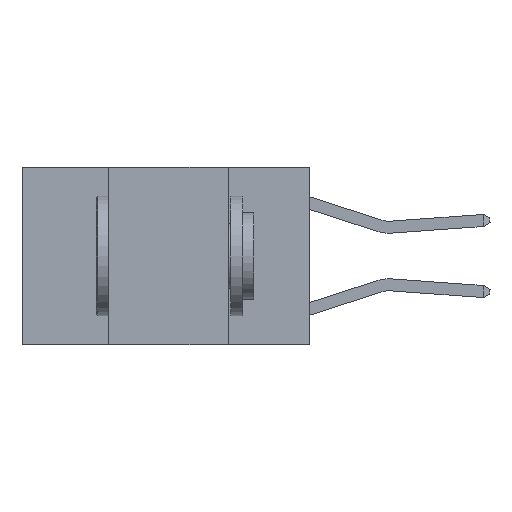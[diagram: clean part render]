
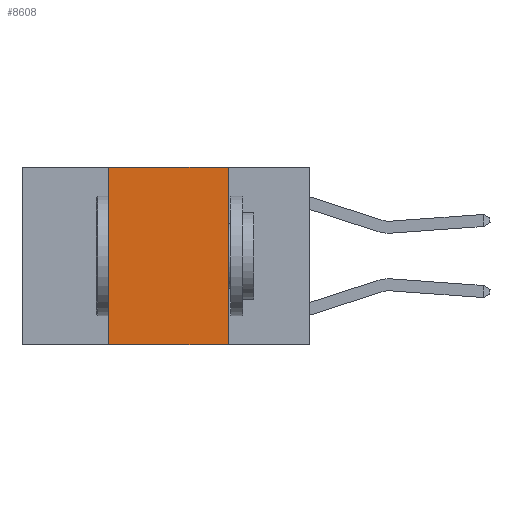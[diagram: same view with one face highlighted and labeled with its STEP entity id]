
A CAD part, left-side view. The second image highlights one B-rep face of the part: STEP entity #8608.
In plain terms, the highlighted planar face has unit normal (-1, 0, 0).
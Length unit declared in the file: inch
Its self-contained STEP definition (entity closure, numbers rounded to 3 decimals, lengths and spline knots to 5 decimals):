
#95 = DIRECTION ( 'NONE',  ( 0., 0., -1. ) ) ;
#164 = CARTESIAN_POINT ( 'NONE',  ( 0., 0.6, 0. ) ) ;
#431 = EDGE_CURVE ( 'NONE', #6142, #10947, #8423, .T. ) ;
#1321 = EDGE_CURVE ( 'NONE', #11035, #5019, #3685, .T. ) ;
#1368 = CARTESIAN_POINT ( 'NONE',  ( 0., 0.17, -0.37 ) ) ;
#1406 = VECTOR ( 'NONE', #2268, 39.37008 ) ;
#1787 = CARTESIAN_POINT ( 'NONE',  ( 0., 0.42, -0.37 ) ) ;
#2268 = DIRECTION ( 'NONE',  ( 0., -1., 0. ) ) ;
#3025 = PLANE ( 'NONE',  #12605 ) ;
#3685 = LINE ( 'NONE', #6578, #8866 ) ;
#5019 = VERTEX_POINT ( 'NONE', #12165 ) ;
#5372 = CARTESIAN_POINT ( 'NONE',  ( 0., 0.6, -0.37 ) ) ;
#5395 = ORIENTED_EDGE ( 'NONE', *, *, #9690, .F. ) ;
#6142 = VERTEX_POINT ( 'NONE', #11469 ) ;
#6363 = ORIENTED_EDGE ( 'NONE', *, *, #431, .F. ) ;
#6578 = CARTESIAN_POINT ( 'NONE',  ( 0., 0.42, 0. ) ) ;
#7197 = CARTESIAN_POINT ( 'NONE',  ( 0., 0.6, 0. ) ) ;
#7323 = DIRECTION ( 'NONE',  ( 0., 0., -1. ) ) ;
#7504 = DIRECTION ( 'NONE',  ( 1., 0., 0. ) ) ;
#7535 = LINE ( 'NONE', #5372, #1406 ) ;
#7894 = DIRECTION ( 'NONE',  ( 0., 0., 1. ) ) ;
#8423 = LINE ( 'NONE', #12596, #9033 ) ;
#8608 = ADVANCED_FACE ( 'NONE', ( #11325 ), #3025, .F. ) ;
#8866 = VECTOR ( 'NONE', #7894, 39.37008 ) ;
#9033 = VECTOR ( 'NONE', #7323, 39.37008 ) ;
#9266 = ORIENTED_EDGE ( 'NONE', *, *, #1321, .F. ) ;
#9690 = EDGE_CURVE ( 'NONE', #5019, #6142, #12489, .T. ) ;
#10722 = DIRECTION ( 'NONE',  ( 0., -1., 0. ) ) ;
#10947 = VERTEX_POINT ( 'NONE', #1368 ) ;
#11035 = VERTEX_POINT ( 'NONE', #1787 ) ;
#11325 = FACE_OUTER_BOUND ( 'NONE', #13384, .T. ) ;
#11469 = CARTESIAN_POINT ( 'NONE',  ( 0., 0.17, 0. ) ) ;
#12165 = CARTESIAN_POINT ( 'NONE',  ( 0., 0.42, 0. ) ) ;
#12489 = LINE ( 'NONE', #7197, #12873 ) ;
#12596 = CARTESIAN_POINT ( 'NONE',  ( 0., 0.17, 0. ) ) ;
#12605 = AXIS2_PLACEMENT_3D ( 'NONE', #164, #7504, #95 ) ;
#12873 = VECTOR ( 'NONE', #10722, 39.37008 ) ;
#13019 = EDGE_CURVE ( 'NONE', #11035, #10947, #7535, .T. ) ;
#13084 = ORIENTED_EDGE ( 'NONE', *, *, #13019, .T. ) ;
#13384 = EDGE_LOOP ( 'NONE', ( #6363, #5395, #9266, #13084 ) ) ;
